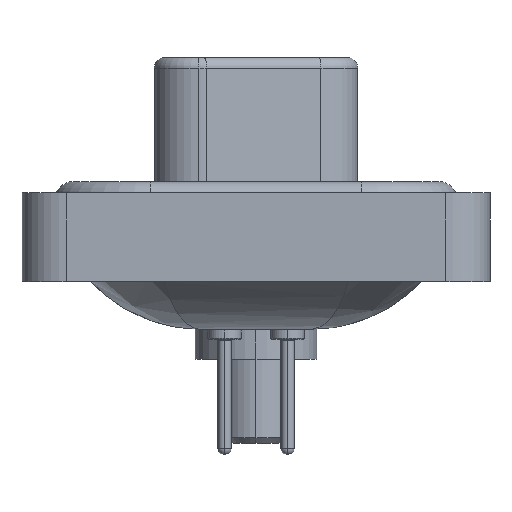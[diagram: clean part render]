
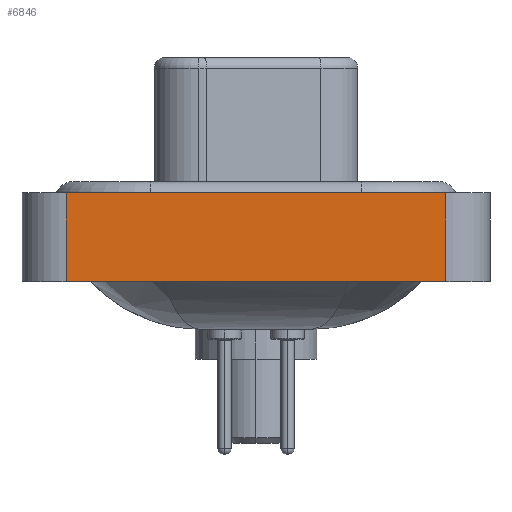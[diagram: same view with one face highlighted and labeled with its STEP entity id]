
A CAD part, left-side view. The second image highlights one B-rep face of the part: STEP entity #6846.
In plain terms, the highlighted planar face has unit normal (-1, 0, 0).
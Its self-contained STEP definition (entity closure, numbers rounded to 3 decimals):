
#270 = DIRECTION ( 'NONE',  ( -1., 0., 0. ) ) ;
#727 = DIRECTION ( 'NONE',  ( 0., -1., 0. ) ) ;
#1360 = LINE ( 'NONE', #13728, #13529 ) ;
#1364 = ORIENTED_EDGE ( 'NONE', *, *, #5999, .T. ) ;
#1540 = CARTESIAN_POINT ( 'NONE',  ( -7.25, 8.55, -3.6 ) ) ;
#2980 = EDGE_LOOP ( 'NONE', ( #5327, #12949, #13823, #1364 ) ) ;
#3685 = LINE ( 'NONE', #9190, #17010 ) ;
#4232 = EDGE_CURVE ( 'NONE', #9738, #11117, #3685, .T. ) ;
#4441 = LINE ( 'NONE', #10036, #6213 ) ;
#5327 = ORIENTED_EDGE ( 'NONE', *, *, #10578, .T. ) ;
#5999 = EDGE_CURVE ( 'NONE', #10666, #6772, #13962, .T. ) ;
#6213 = VECTOR ( 'NONE', #9955, 1000. ) ;
#6772 = VERTEX_POINT ( 'NONE', #10919 ) ;
#6846 = ADVANCED_FACE ( 'NONE', ( #7205 ), #7110, .T. ) ;
#7110 = PLANE ( 'NONE',  #9277 ) ;
#7205 = FACE_OUTER_BOUND ( 'NONE', #2980, .T. ) ;
#8033 = DIRECTION ( 'NONE',  ( 0., 0., 1. ) ) ;
#8108 = EDGE_CURVE ( 'NONE', #10666, #9738, #4441, .T. ) ;
#8550 = DIRECTION ( 'NONE',  ( 0., -1., 0. ) ) ;
#9190 = CARTESIAN_POINT ( 'NONE',  ( -7.25, -8.55, 0.4 ) ) ;
#9277 = AXIS2_PLACEMENT_3D ( 'NONE', #11191, #270, #11292 ) ;
#9718 = CARTESIAN_POINT ( 'NONE',  ( -7.25, -8.55, -3.6 ) ) ;
#9738 = VERTEX_POINT ( 'NONE', #16477 ) ;
#9955 = DIRECTION ( 'NONE',  ( 0., 0., 1. ) ) ;
#9983 = CARTESIAN_POINT ( 'NONE',  ( -7.25, -8.55, 0.4 ) ) ;
#10036 = CARTESIAN_POINT ( 'NONE',  ( -7.25, 8.55, -3.6 ) ) ;
#10578 = EDGE_CURVE ( 'NONE', #6772, #11117, #1360, .T. ) ;
#10666 = VERTEX_POINT ( 'NONE', #1540 ) ;
#10919 = CARTESIAN_POINT ( 'NONE',  ( -7.25, -8.55, -3.6 ) ) ;
#11117 = VERTEX_POINT ( 'NONE', #9983 ) ;
#11191 = CARTESIAN_POINT ( 'NONE',  ( -7.25, -8.55, -3.6 ) ) ;
#11292 = DIRECTION ( 'NONE',  ( 0., 0., 1. ) ) ;
#12949 = ORIENTED_EDGE ( 'NONE', *, *, #4232, .F. ) ;
#13529 = VECTOR ( 'NONE', #8033, 1000. ) ;
#13728 = CARTESIAN_POINT ( 'NONE',  ( -7.25, -8.55, -3.6 ) ) ;
#13823 = ORIENTED_EDGE ( 'NONE', *, *, #8108, .F. ) ;
#13962 = LINE ( 'NONE', #9718, #14716 ) ;
#14716 = VECTOR ( 'NONE', #8550, 1000. ) ;
#16477 = CARTESIAN_POINT ( 'NONE',  ( -7.25, 8.55, 0.4 ) ) ;
#17010 = VECTOR ( 'NONE', #727, 1000. ) ;
